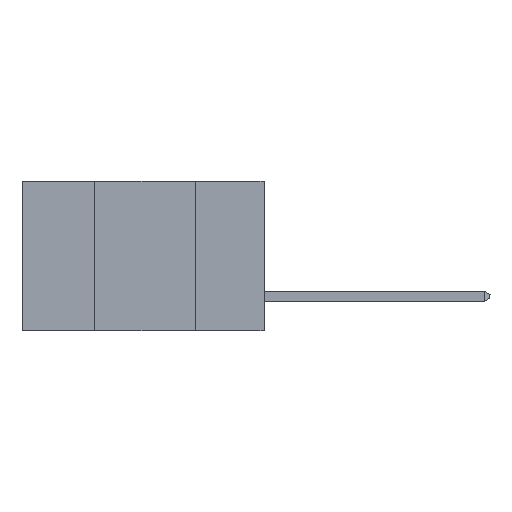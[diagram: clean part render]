
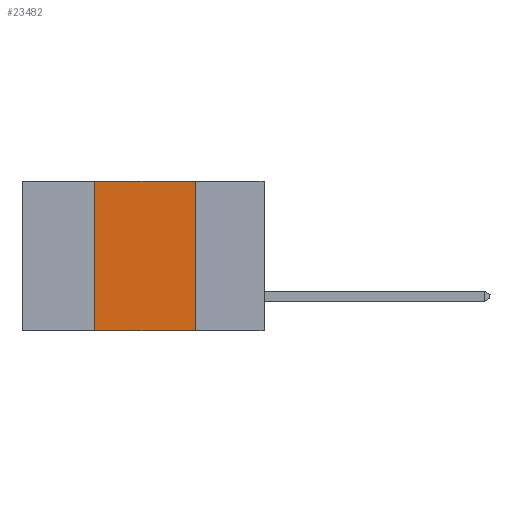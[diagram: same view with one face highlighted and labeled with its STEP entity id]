
A CAD part, left-side view. The second image highlights one B-rep face of the part: STEP entity #23482.
In plain terms, the highlighted planar face has unit normal (-1, 0, 0).
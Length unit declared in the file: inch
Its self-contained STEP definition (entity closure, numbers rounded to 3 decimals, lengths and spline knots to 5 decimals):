
#347 = VERTEX_POINT ( 'NONE', #10667 ) ;
#620 = CARTESIAN_POINT ( 'NONE',  ( 0., 0.6, 0. ) ) ;
#789 = PLANE ( 'NONE',  #16462 ) ;
#905 = ORIENTED_EDGE ( 'NONE', *, *, #10544, .T. ) ;
#1684 = DIRECTION ( 'NONE',  ( 0., -1., 0. ) ) ;
#2191 = EDGE_CURVE ( 'NONE', #11061, #3769, #10075, .T. ) ;
#2774 = ORIENTED_EDGE ( 'NONE', *, *, #2191, .F. ) ;
#3034 = EDGE_CURVE ( 'NONE', #3769, #347, #22261, .T. ) ;
#3140 = CARTESIAN_POINT ( 'NONE',  ( 0., 0.17, 0. ) ) ;
#3769 = VERTEX_POINT ( 'NONE', #25276 ) ;
#4147 = ORIENTED_EDGE ( 'NONE', *, *, #3034, .F. ) ;
#7390 = LINE ( 'NONE', #9897, #8959 ) ;
#7978 = DIRECTION ( 'NONE',  ( 0., 0., 1. ) ) ;
#8959 = VECTOR ( 'NONE', #7978, 39.37008 ) ;
#9897 = CARTESIAN_POINT ( 'NONE',  ( 0., 0.42, 0. ) ) ;
#10075 = LINE ( 'NONE', #11486, #22283 ) ;
#10544 = EDGE_CURVE ( 'NONE', #14060, #347, #18550, .T. ) ;
#10667 = CARTESIAN_POINT ( 'NONE',  ( 0., 0.17, -0.37 ) ) ;
#11061 = VERTEX_POINT ( 'NONE', #23171 ) ;
#11486 = CARTESIAN_POINT ( 'NONE',  ( 0., 0.6, 0. ) ) ;
#11543 = CARTESIAN_POINT ( 'NONE',  ( 0., 0.6, -0.37 ) ) ;
#11955 = ORIENTED_EDGE ( 'NONE', *, *, #15625, .F. ) ;
#12660 = DIRECTION ( 'NONE',  ( 1., 0., 0. ) ) ;
#14060 = VERTEX_POINT ( 'NONE', #18145 ) ;
#14449 = VECTOR ( 'NONE', #25531, 39.37008 ) ;
#14552 = FACE_OUTER_BOUND ( 'NONE', #16226, .T. ) ;
#15625 = EDGE_CURVE ( 'NONE', #14060, #11061, #7390, .T. ) ;
#16226 = EDGE_LOOP ( 'NONE', ( #4147, #2774, #11955, #905 ) ) ;
#16462 = AXIS2_PLACEMENT_3D ( 'NONE', #620, #12660, #20725 ) ;
#17165 = DIRECTION ( 'NONE',  ( 0., 0., -1. ) ) ;
#18145 = CARTESIAN_POINT ( 'NONE',  ( 0., 0.42, -0.37 ) ) ;
#18550 = LINE ( 'NONE', #11543, #14449 ) ;
#20725 = DIRECTION ( 'NONE',  ( 0., 0., -1. ) ) ;
#22261 = LINE ( 'NONE', #3140, #25391 ) ;
#22283 = VECTOR ( 'NONE', #1684, 39.37008 ) ;
#23171 = CARTESIAN_POINT ( 'NONE',  ( 0., 0.42, 0. ) ) ;
#23482 = ADVANCED_FACE ( 'NONE', ( #14552 ), #789, .F. ) ;
#25276 = CARTESIAN_POINT ( 'NONE',  ( 0., 0.17, 0. ) ) ;
#25391 = VECTOR ( 'NONE', #17165, 39.37008 ) ;
#25531 = DIRECTION ( 'NONE',  ( 0., -1., 0. ) ) ;
